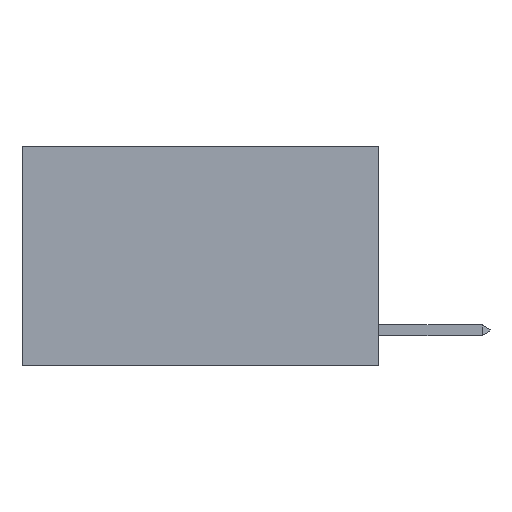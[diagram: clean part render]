
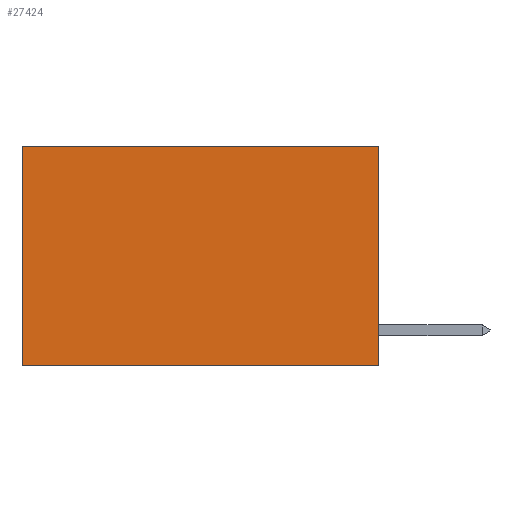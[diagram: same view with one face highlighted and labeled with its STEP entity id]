
A CAD part, left-side view. The second image highlights one B-rep face of the part: STEP entity #27424.
In plain terms, the highlighted planar face has unit normal (-1, 0, 0).
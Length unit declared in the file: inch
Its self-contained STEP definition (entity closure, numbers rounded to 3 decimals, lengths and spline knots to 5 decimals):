
#2848 = CARTESIAN_POINT ( 'NONE',  ( 0.2625, 0.6, 0. ) ) ;
#3092 = AXIS2_PLACEMENT_3D ( 'NONE', #27811, #16742, #3511 ) ;
#3511 = DIRECTION ( 'NONE',  ( 0., 0., -1. ) ) ;
#4928 = EDGE_CURVE ( 'NONE', #8883, #7203, #17337, .T. ) ;
#7203 = VERTEX_POINT ( 'NONE', #17551 ) ;
#7387 = DIRECTION ( 'NONE',  ( 0., 1., 0. ) ) ;
#8883 = VERTEX_POINT ( 'NONE', #11159 ) ;
#9370 = EDGE_CURVE ( 'NONE', #28426, #21335, #17794, .T. ) ;
#10179 = CARTESIAN_POINT ( 'NONE',  ( 0.2625, 0.6, 0. ) ) ;
#11159 = CARTESIAN_POINT ( 'NONE',  ( 0.2625, 0., 0. ) ) ;
#11707 = CARTESIAN_POINT ( 'NONE',  ( 0.2625, 0., -0.37 ) ) ;
#11765 = CARTESIAN_POINT ( 'NONE',  ( 0.2625, 0., 0. ) ) ;
#12332 = PLANE ( 'NONE',  #3092 ) ;
#12648 = EDGE_LOOP ( 'NONE', ( #18001, #23842, #24539, #20091 ) ) ;
#13804 = LINE ( 'NONE', #11707, #25504 ) ;
#14206 = EDGE_CURVE ( 'NONE', #8883, #28426, #26567, .T. ) ;
#14598 = DIRECTION ( 'NONE',  ( 0., 0., -1. ) ) ;
#15133 = FACE_OUTER_BOUND ( 'NONE', #12648, .T. ) ;
#16097 = CARTESIAN_POINT ( 'NONE',  ( 0.2625, 0., 0. ) ) ;
#16742 = DIRECTION ( 'NONE',  ( 1., 0., 0. ) ) ;
#17337 = LINE ( 'NONE', #11765, #27046 ) ;
#17551 = CARTESIAN_POINT ( 'NONE',  ( 0.2625, 0., -0.37 ) ) ;
#17794 = LINE ( 'NONE', #10179, #22919 ) ;
#18001 = ORIENTED_EDGE ( 'NONE', *, *, #9370, .T. ) ;
#19842 = CARTESIAN_POINT ( 'NONE',  ( 0.2625, 0.6, -0.37 ) ) ;
#19986 = VECTOR ( 'NONE', #7387, 39.37008 ) ;
#20091 = ORIENTED_EDGE ( 'NONE', *, *, #14206, .T. ) ;
#21335 = VERTEX_POINT ( 'NONE', #19842 ) ;
#22919 = VECTOR ( 'NONE', #14598, 39.37008 ) ;
#23842 = ORIENTED_EDGE ( 'NONE', *, *, #26673, .F. ) ;
#24539 = ORIENTED_EDGE ( 'NONE', *, *, #4928, .F. ) ;
#24907 = DIRECTION ( 'NONE',  ( 0., 0., -1. ) ) ;
#25504 = VECTOR ( 'NONE', #27143, 39.37008 ) ;
#26567 = LINE ( 'NONE', #16097, #19986 ) ;
#26673 = EDGE_CURVE ( 'NONE', #7203, #21335, #13804, .T. ) ;
#27046 = VECTOR ( 'NONE', #24907, 39.37008 ) ;
#27143 = DIRECTION ( 'NONE',  ( 0., 1., 0. ) ) ;
#27424 = ADVANCED_FACE ( 'NONE', ( #15133 ), #12332, .F. ) ;
#27811 = CARTESIAN_POINT ( 'NONE',  ( 0.2625, 0., 0. ) ) ;
#28426 = VERTEX_POINT ( 'NONE', #2848 ) ;
